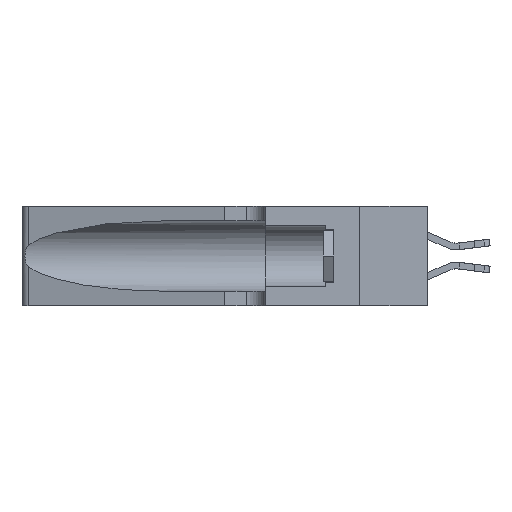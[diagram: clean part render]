
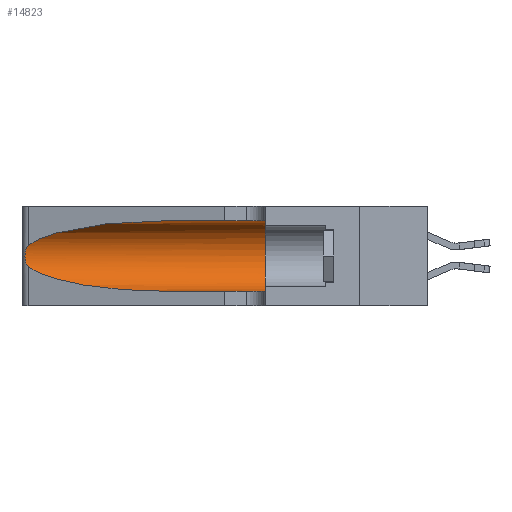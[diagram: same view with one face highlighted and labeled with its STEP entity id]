
A CAD part, left-side view. The second image highlights one B-rep face of the part: STEP entity #14823.
In plain terms, the highlighted cylindrical face has radius 3.308 mm (diameter 6.617 mm), a partial arc.
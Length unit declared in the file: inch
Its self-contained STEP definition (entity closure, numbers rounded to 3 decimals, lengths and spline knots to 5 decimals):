
#1039 = CARTESIAN_POINT ( 'NONE',  ( 0.25487, 1.22718, 0.14631 ) ) ;
#1311 = ORIENTED_EDGE ( 'NONE', *, *, #31530, .T. ) ;
#1618 = AXIS2_PLACEMENT_3D ( 'NONE', #15553, #35244, #18401 ) ;
#2320 = VERTEX_POINT ( 'NONE', #15932 ) ;
#2375 = CARTESIAN_POINT ( 'NONE',  ( 0.25555, 1.22994, 0.2215 ) ) ;
#2497 = CARTESIAN_POINT ( 'NONE',  ( 0.25639, 1.23186, 0.15144 ) ) ;
#3967 = ORIENTED_EDGE ( 'NONE', *, *, #20216, .F. ) ;
#4415 = ORIENTED_EDGE ( 'NONE', *, *, #24516, .F. ) ;
#5220 = DIRECTION ( 'NONE',  ( 0., -1., 0. ) ) ;
#5297 = CARTESIAN_POINT ( 'NONE',  ( 0.25487, 1.22718, 0.22369 ) ) ;
#5411 = VECTOR ( 'NONE', #21231, 39.37008 ) ;
#5420 = CARTESIAN_POINT ( 'NONE',  ( 0.25487, 1.22718, 0.14631 ) ) ;
#5753 = CARTESIAN_POINT ( 'NONE',  ( 0.25487, 1.22718, 0.22369 ) ) ;
#5910 = EDGE_CURVE ( 'NONE', #30382, #2320, #35099, .T. ) ;
#6165 = VERTEX_POINT ( 'NONE', #1039 ) ;
#8184 = CARTESIAN_POINT ( 'NONE',  ( 0.25639, 1.23184, 0.21858 ) ) ;
#8855 = CARTESIAN_POINT ( 'NONE',  ( 0.1305, 0.35, 0.05475 ) ) ;
#9078 = CARTESIAN_POINT ( 'NONE',  ( 0.1305, 0.72297, 0.31525 ) ) ;
#9563 = CARTESIAN_POINT ( 'NONE',  ( 0.25487, 1.22718, 0.14631 ) ) ;
#9992 = B_SPLINE_CURVE_WITH_KNOTS ( 'NONE', 3,
 ( #5297, #2375, #8184, #27972, #11036, #30818, #13903, #33618, #16772, #36434, #19606, #2497, #22428, #5420 ),
 .UNSPECIFIED., .F., .F.,
 ( 4, 2, 2, 2, 2, 2, 4 ),
 ( 0., 0.00027, 0.00053, 0.00107, 0.0016, 0.00187, 0.00214 ),
 .UNSPECIFIED. ) ;
#10390 = AXIS2_PLACEMENT_3D ( 'NONE', #22237, #5220, #30750 ) ;
#11036 = CARTESIAN_POINT ( 'NONE',  ( 0.25854, 1.2359, 0.20912 ) ) ;
#11375 = CARTESIAN_POINT ( 'NONE',  ( 0.18966, 0.96281, 0.31525 ) ) ;
#11555 = ORIENTED_EDGE ( 'NONE', *, *, #28970, .T. ) ;
#12520 = CYLINDRICAL_SURFACE ( 'NONE', #10390, 0.13025 ) ;
#13903 = CARTESIAN_POINT ( 'NONE',  ( 0.26075, 1.23896, 0.19203 ) ) ;
#14823 = ADVANCED_FACE ( 'NONE', ( #21840 ), #12520, .F. ) ;
#15242 = ORIENTED_EDGE ( 'NONE', *, *, #5910, .T. ) ;
#15302 = CARTESIAN_POINT ( 'NONE',  ( 0.1305, 0.72297, 0.05475 ) ) ;
#15553 = CARTESIAN_POINT ( 'NONE',  ( 0.1305, 0.35, 0.185 ) ) ;
#15932 = CARTESIAN_POINT ( 'NONE',  ( 0.25487, 1.22718, 0.22369 ) ) ;
#16635 = LINE ( 'NONE', #26686, #23234 ) ;
#16772 = CARTESIAN_POINT ( 'NONE',  ( 0.26017, 1.23833, 0.17102 ) ) ;
#17808 = EDGE_LOOP ( 'NONE', ( #15242, #11555, #1311, #30645, #4415, #3967 ) ) ;
#18401 = DIRECTION ( 'NONE',  ( 0., 0., 1. ) ) ;
#18434 = CARTESIAN_POINT ( 'NONE',  ( 0.1305, 1.61858, 0.31525 ) ) ;
#19606 = CARTESIAN_POINT ( 'NONE',  ( 0.25789, 1.23486, 0.15765 ) ) ;
#20216 = EDGE_CURVE ( 'NONE', #30382, #35929, #35514, .T. ) ;
#21231 = DIRECTION ( 'NONE',  ( 0., -1., 0. ) ) ;
#21840 = FACE_OUTER_BOUND ( 'NONE', #17808, .T. ) ;
#22237 = CARTESIAN_POINT ( 'NONE',  ( 0.1305, 1.61858, 0.185 ) ) ;
#22428 = CARTESIAN_POINT ( 'NONE',  ( 0.25555, 1.22993, 0.14849 ) ) ;
#22759 = CARTESIAN_POINT ( 'NONE',  ( 0.2373, 1.15595, 0.28018 ) ) ;
#23234 = VECTOR ( 'NONE', #29545, 39.37008 ) ;
#24516 = EDGE_CURVE ( 'NONE', #35929, #32730, #24697, .T. ) ;
#24566 = CARTESIAN_POINT ( 'NONE',  ( 0.1305, 0.72297, 0.05475 ) ) ;
#24697 = CIRCLE ( 'NONE', #1618, 0.13025 ) ;
#26686 = CARTESIAN_POINT ( 'NONE',  ( 0.1305, 1.61858, 0.05475 ) ) ;
#26817 = EDGE_CURVE ( 'NONE', #35870, #32730, #16635, .T. ) ;
#27735 = CARTESIAN_POINT ( 'NONE',  ( 0.1305, 0.35, 0.31525 ) ) ;
#27972 = CARTESIAN_POINT ( 'NONE',  ( 0.25787, 1.23484, 0.2124 ) ) ;
#28970 = EDGE_CURVE ( 'NONE', #2320, #6165, #9992, .T. ) ;
#29351 = CARTESIAN_POINT ( 'NONE',  ( 0.2373, 1.15595, 0.08982 ) ) ;
#29545 = DIRECTION ( 'NONE',  ( 0., -1., 0. ) ) ;
#30382 = VERTEX_POINT ( 'NONE', #9078 ) ;
#30645 = ORIENTED_EDGE ( 'NONE', *, *, #26817, .T. ) ;
#30750 = DIRECTION ( 'NONE',  ( 0., 0., -1. ) ) ;
#30818 = CARTESIAN_POINT ( 'NONE',  ( 0.26018, 1.23835, 0.19895 ) ) ;
#31159 = CARTESIAN_POINT ( 'NONE',  ( 0.1305, 0.72297, 0.31525 ) ) ;
#31530 = EDGE_CURVE ( 'NONE', #6165, #35870, #33518, .T. ) ;
#32180 = CARTESIAN_POINT ( 'NONE',  ( 0.18966, 0.96281, 0.05475 ) ) ;
#32730 = VERTEX_POINT ( 'NONE', #8855 ) ;
#33518 =( BOUNDED_CURVE ( )  B_SPLINE_CURVE ( 3, ( #9563, #29351, #32180, #15302 ),
 .UNSPECIFIED., .F., .F. ) 
 B_SPLINE_CURVE_WITH_KNOTS ( ( 4, 4 ),
 ( 3.44316, 4.71239 ),
 .UNSPECIFIED. ) 
 CURVE ( )  GEOMETRIC_REPRESENTATION_ITEM ( )  RATIONAL_B_SPLINE_CURVE ( ( 1., 0.87, 0.87, 1. ) ) 
 REPRESENTATION_ITEM ( '' )  );
#33618 = CARTESIAN_POINT ( 'NONE',  ( 0.26075, 1.23896, 0.178 ) ) ;
#35099 =( BOUNDED_CURVE ( )  B_SPLINE_CURVE ( 3, ( #31159, #11375, #22759, #5753 ),
 .UNSPECIFIED., .F., .T. ) 
 B_SPLINE_CURVE_WITH_KNOTS ( ( 4, 4 ),
 ( 1.5708, 2.84003 ),
 .UNSPECIFIED. ) 
 CURVE ( )  GEOMETRIC_REPRESENTATION_ITEM ( )  RATIONAL_B_SPLINE_CURVE ( ( 1., 0.87, 0.87, 1. ) ) 
 REPRESENTATION_ITEM ( '' )  );
#35244 = DIRECTION ( 'NONE',  ( 0., 1., 0. ) ) ;
#35514 = LINE ( 'NONE', #18434, #5411 ) ;
#35870 = VERTEX_POINT ( 'NONE', #24566 ) ;
#35929 = VERTEX_POINT ( 'NONE', #27735 ) ;
#36434 = CARTESIAN_POINT ( 'NONE',  ( 0.25856, 1.23593, 0.16098 ) ) ;
